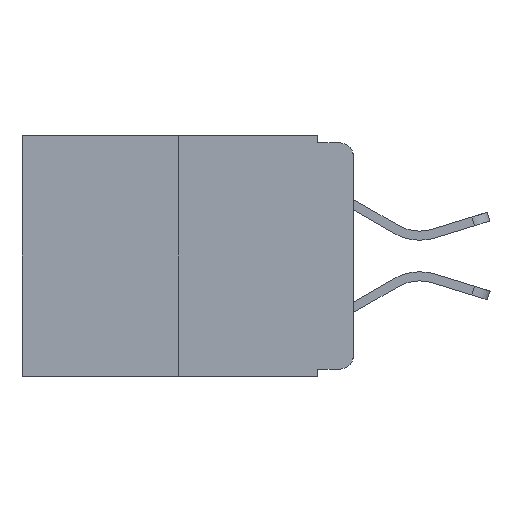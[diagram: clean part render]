
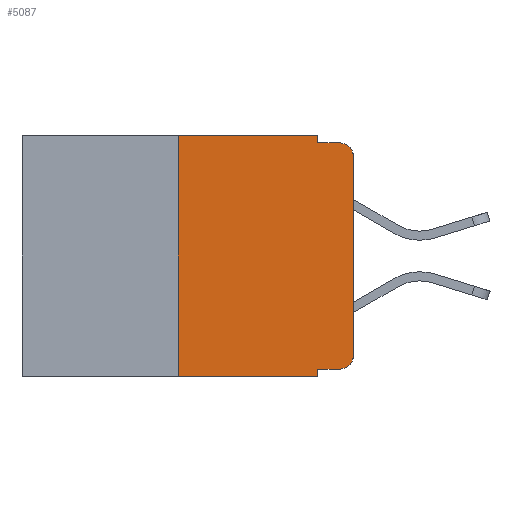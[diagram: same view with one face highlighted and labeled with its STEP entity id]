
A CAD part, left-side view. The second image highlights one B-rep face of the part: STEP entity #5087.
In plain terms, the highlighted planar face has unit normal (-1, 0, 0).
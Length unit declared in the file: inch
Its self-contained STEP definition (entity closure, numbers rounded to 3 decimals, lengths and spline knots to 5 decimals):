
#243 = CARTESIAN_POINT ( 'NONE',  ( 0., 0.473, 0. ) ) ;
#528 = FACE_OUTER_BOUND ( 'NONE', #14468, .T. ) ;
#1243 = CIRCLE ( 'NONE', #7709, 0.02 ) ;
#1412 = ORIENTED_EDGE ( 'NONE', *, *, #20451, .F. ) ;
#1807 = VECTOR ( 'NONE', #16345, 39.37008 ) ;
#2286 = CARTESIAN_POINT ( 'NONE',  ( 0., 0.473, -0.343 ) ) ;
#2377 = VERTEX_POINT ( 'NONE', #12708 ) ;
#3063 = ORIENTED_EDGE ( 'NONE', *, *, #7380, .T. ) ;
#3084 = VERTEX_POINT ( 'NONE', #13908 ) ;
#3102 = CARTESIAN_POINT ( 'NONE',  ( 0., 0.051, 0. ) ) ;
#3217 = CARTESIAN_POINT ( 'NONE',  ( 0., 0.051, -0.01 ) ) ;
#3400 = EDGE_CURVE ( 'NONE', #17745, #10065, #6873, .T. ) ;
#3538 = DIRECTION ( 'NONE',  ( 0., -1., 0. ) ) ;
#3702 = CARTESIAN_POINT ( 'NONE',  ( 0., 0.051, -0.333 ) ) ;
#3787 = DIRECTION ( 'NONE',  ( 0., 0., -1. ) ) ;
#3893 = LINE ( 'NONE', #7077, #10336 ) ;
#4135 = CARTESIAN_POINT ( 'NONE',  ( 0., 0.25, 0. ) ) ;
#4336 = LINE ( 'NONE', #4135, #5414 ) ;
#4880 = VECTOR ( 'NONE', #18663, 39.37008 ) ;
#5087 = ADVANCED_FACE ( 'NONE', ( #528 ), #16694, .F. ) ;
#5284 = VECTOR ( 'NONE', #19940, 39.37008 ) ;
#5414 = VECTOR ( 'NONE', #14014, 39.37008 ) ;
#5754 = EDGE_CURVE ( 'NONE', #17554, #9611, #10149, .T. ) ;
#6671 = ORIENTED_EDGE ( 'NONE', *, *, #13667, .T. ) ;
#6850 = CARTESIAN_POINT ( 'NONE',  ( 0., 0.02, -0.313 ) ) ;
#6873 = LINE ( 'NONE', #3702, #1807 ) ;
#7077 = CARTESIAN_POINT ( 'NONE',  ( 0., 0.051, 0. ) ) ;
#7109 = EDGE_CURVE ( 'NONE', #17745, #3084, #3893, .T. ) ;
#7242 = CARTESIAN_POINT ( 'NONE',  ( 0., 0.051, -0.01 ) ) ;
#7380 = EDGE_CURVE ( 'NONE', #17460, #2377, #1243, .T. ) ;
#7621 = ORIENTED_EDGE ( 'NONE', *, *, #14817, .F. ) ;
#7709 = AXIS2_PLACEMENT_3D ( 'NONE', #12963, #16178, #9506 ) ;
#7780 = CARTESIAN_POINT ( 'NONE',  ( 0., 0.25, 0. ) ) ;
#8636 = DIRECTION ( 'NONE',  ( 1., 0., 0. ) ) ;
#8744 = CARTESIAN_POINT ( 'NONE',  ( 0., 0.473, 0. ) ) ;
#8808 = ORIENTED_EDGE ( 'NONE', *, *, #11745, .T. ) ;
#9506 = DIRECTION ( 'NONE',  ( 0., 0., -1. ) ) ;
#9606 = DIRECTION ( 'NONE',  ( 0., 0., -1. ) ) ;
#9611 = VERTEX_POINT ( 'NONE', #12418 ) ;
#10065 = VERTEX_POINT ( 'NONE', #17179 ) ;
#10149 = LINE ( 'NONE', #243, #5284 ) ;
#10312 = VECTOR ( 'NONE', #3538, 39.37008 ) ;
#10330 = DIRECTION ( 'NONE',  ( 0., 0., -1. ) ) ;
#10336 = VECTOR ( 'NONE', #3787, 39.37008 ) ;
#11724 = AXIS2_PLACEMENT_3D ( 'NONE', #8744, #8636, #10330 ) ;
#11733 = ORIENTED_EDGE ( 'NONE', *, *, #17962, .T. ) ;
#11745 = EDGE_CURVE ( 'NONE', #19309, #3084, #12173, .T. ) ;
#11882 = AXIS2_PLACEMENT_3D ( 'NONE', #6850, #16535, #21013 ) ;
#12173 = LINE ( 'NONE', #2286, #4880 ) ;
#12418 = CARTESIAN_POINT ( 'NONE',  ( 0., 0.051, 0. ) ) ;
#12474 = VERTEX_POINT ( 'NONE', #15045 ) ;
#12708 = CARTESIAN_POINT ( 'NONE',  ( 0., 0.02, -0.01 ) ) ;
#12963 = CARTESIAN_POINT ( 'NONE',  ( 0., 0.02, -0.03 ) ) ;
#13114 = ORIENTED_EDGE ( 'NONE', *, *, #17540, .F. ) ;
#13667 = EDGE_CURVE ( 'NONE', #10065, #12474, #18872, .T. ) ;
#13908 = CARTESIAN_POINT ( 'NONE',  ( 0., 0.051, -0.343 ) ) ;
#14014 = DIRECTION ( 'NONE',  ( 0., 0., 1. ) ) ;
#14468 = EDGE_LOOP ( 'NONE', ( #11733, #3063, #1412, #13114, #16214, #7621, #8808, #17712, #16643, #6671 ) ) ;
#14817 = EDGE_CURVE ( 'NONE', #19309, #17554, #4336, .T. ) ;
#14907 = LINE ( 'NONE', #3217, #10312 ) ;
#15045 = CARTESIAN_POINT ( 'NONE',  ( 0., 0., -0.313 ) ) ;
#15548 = CARTESIAN_POINT ( 'NONE',  ( 0., 0., -0.03 ) ) ;
#16178 = DIRECTION ( 'NONE',  ( -1., 0., 0. ) ) ;
#16214 = ORIENTED_EDGE ( 'NONE', *, *, #5754, .F. ) ;
#16345 = DIRECTION ( 'NONE',  ( 0., -1., 0. ) ) ;
#16535 = DIRECTION ( 'NONE',  ( -1., 0., 0. ) ) ;
#16643 = ORIENTED_EDGE ( 'NONE', *, *, #3400, .T. ) ;
#16694 = PLANE ( 'NONE',  #11724 ) ;
#17039 = VECTOR ( 'NONE', #9606, 39.37008 ) ;
#17179 = CARTESIAN_POINT ( 'NONE',  ( 0., 0.02, -0.333 ) ) ;
#17332 = DIRECTION ( 'NONE',  ( 0., 0., 1. ) ) ;
#17460 = VERTEX_POINT ( 'NONE', #15548 ) ;
#17540 = EDGE_CURVE ( 'NONE', #9611, #20498, #17667, .T. ) ;
#17554 = VERTEX_POINT ( 'NONE', #7780 ) ;
#17643 = CARTESIAN_POINT ( 'NONE',  ( 0., 0., 0. ) ) ;
#17667 = LINE ( 'NONE', #3102, #17039 ) ;
#17712 = ORIENTED_EDGE ( 'NONE', *, *, #7109, .F. ) ;
#17745 = VERTEX_POINT ( 'NONE', #19590 ) ;
#17962 = EDGE_CURVE ( 'NONE', #12474, #17460, #19353, .T. ) ;
#18663 = DIRECTION ( 'NONE',  ( 0., -1., 0. ) ) ;
#18872 = CIRCLE ( 'NONE', #11882, 0.02 ) ;
#19309 = VERTEX_POINT ( 'NONE', #20425 ) ;
#19353 = LINE ( 'NONE', #17643, #20806 ) ;
#19590 = CARTESIAN_POINT ( 'NONE',  ( 0., 0.051, -0.333 ) ) ;
#19940 = DIRECTION ( 'NONE',  ( 0., -1., 0. ) ) ;
#20425 = CARTESIAN_POINT ( 'NONE',  ( 0., 0.25, -0.343 ) ) ;
#20451 = EDGE_CURVE ( 'NONE', #20498, #2377, #14907, .T. ) ;
#20498 = VERTEX_POINT ( 'NONE', #7242 ) ;
#20806 = VECTOR ( 'NONE', #17332, 39.37008 ) ;
#21013 = DIRECTION ( 'NONE',  ( 0., 0., -1. ) ) ;
